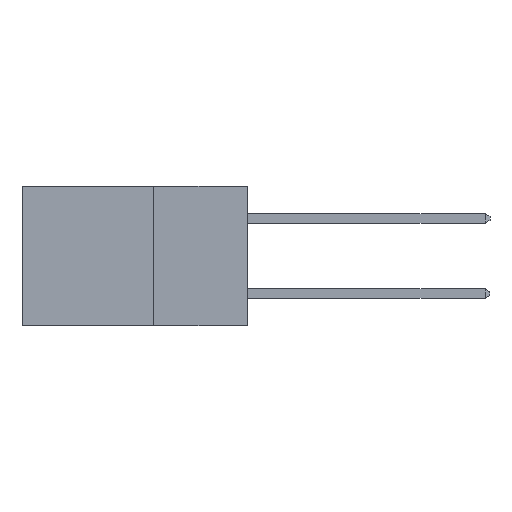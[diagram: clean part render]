
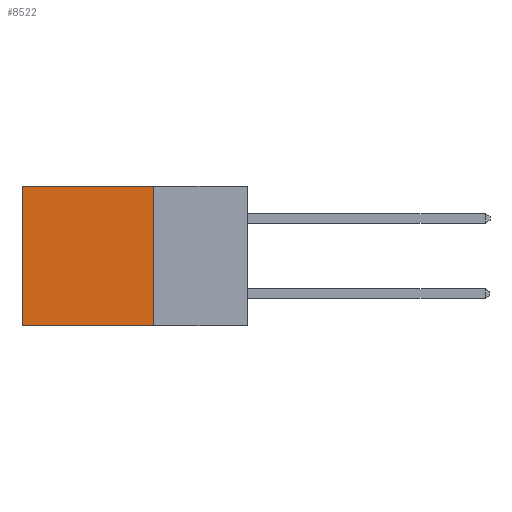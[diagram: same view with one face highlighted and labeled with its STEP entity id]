
A CAD part, left-side view. The second image highlights one B-rep face of the part: STEP entity #8522.
In plain terms, the highlighted planar face has unit normal (-1, 0, 0).
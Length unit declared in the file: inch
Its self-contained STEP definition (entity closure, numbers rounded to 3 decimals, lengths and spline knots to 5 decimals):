
#404 = PLANE ( 'NONE',  #10629 ) ;
#673 = DIRECTION ( 'NONE',  ( 0., 1., 0. ) ) ;
#699 = CARTESIAN_POINT ( 'NONE',  ( 0.298, 0.25, -0.37 ) ) ;
#1004 = VECTOR ( 'NONE', #5349, 39.37008 ) ;
#1436 = VECTOR ( 'NONE', #673, 39.37008 ) ;
#1888 = VECTOR ( 'NONE', #10324, 39.37008 ) ;
#2062 = DIRECTION ( 'NONE',  ( 0., 0., -1. ) ) ;
#2118 = CARTESIAN_POINT ( 'NONE',  ( 0.298, 0.6, 0. ) ) ;
#2184 = DIRECTION ( 'NONE',  ( 0., 0., -1. ) ) ;
#2773 = VERTEX_POINT ( 'NONE', #6615 ) ;
#2835 = FACE_OUTER_BOUND ( 'NONE', #4458, .T. ) ;
#3200 = EDGE_CURVE ( 'NONE', #2773, #4014, #3529, .T. ) ;
#3268 = LINE ( 'NONE', #8047, #1004 ) ;
#3370 = CARTESIAN_POINT ( 'NONE',  ( 0.298, 0.25, 0. ) ) ;
#3487 = VERTEX_POINT ( 'NONE', #9253 ) ;
#3529 = LINE ( 'NONE', #2118, #7678 ) ;
#3549 = EDGE_CURVE ( 'NONE', #9897, #2773, #3268, .T. ) ;
#4014 = VERTEX_POINT ( 'NONE', #6570 ) ;
#4099 = LINE ( 'NONE', #4762, #1888 ) ;
#4281 = ORIENTED_EDGE ( 'NONE', *, *, #3549, .T. ) ;
#4458 = EDGE_LOOP ( 'NONE', ( #8467, #7917, #10003, #4281 ) ) ;
#4762 = CARTESIAN_POINT ( 'NONE',  ( 0.298, 0.25, 0. ) ) ;
#5087 = EDGE_CURVE ( 'NONE', #3487, #4014, #9629, .T. ) ;
#5349 = DIRECTION ( 'NONE',  ( 0., 1., 0. ) ) ;
#6570 = CARTESIAN_POINT ( 'NONE',  ( 0.298, 0.6, -0.37 ) ) ;
#6615 = CARTESIAN_POINT ( 'NONE',  ( 0.298, 0.6, 0. ) ) ;
#7137 = DIRECTION ( 'NONE',  ( 1., 0., 0. ) ) ;
#7678 = VECTOR ( 'NONE', #2062, 39.37008 ) ;
#7917 = ORIENTED_EDGE ( 'NONE', *, *, #5087, .F. ) ;
#8047 = CARTESIAN_POINT ( 'NONE',  ( 0.298, 0.25, 0. ) ) ;
#8467 = ORIENTED_EDGE ( 'NONE', *, *, #3200, .T. ) ;
#8522 = ADVANCED_FACE ( 'NONE', ( #2835 ), #404, .F. ) ;
#9253 = CARTESIAN_POINT ( 'NONE',  ( 0.298, 0.25, -0.37 ) ) ;
#9413 = EDGE_CURVE ( 'NONE', #9897, #3487, #4099, .T. ) ;
#9629 = LINE ( 'NONE', #699, #1436 ) ;
#9897 = VERTEX_POINT ( 'NONE', #3370 ) ;
#10003 = ORIENTED_EDGE ( 'NONE', *, *, #9413, .F. ) ;
#10218 = CARTESIAN_POINT ( 'NONE',  ( 0.298, 0.25, 0. ) ) ;
#10324 = DIRECTION ( 'NONE',  ( 0., 0., -1. ) ) ;
#10629 = AXIS2_PLACEMENT_3D ( 'NONE', #10218, #7137, #2184 ) ;
